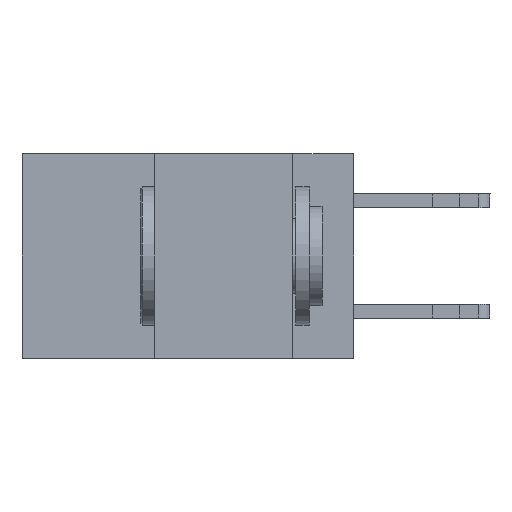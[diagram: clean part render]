
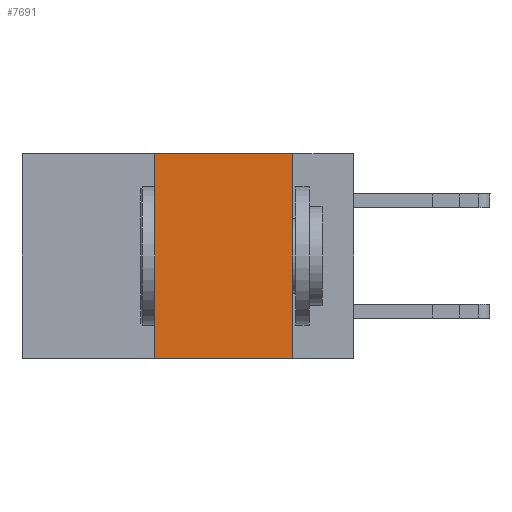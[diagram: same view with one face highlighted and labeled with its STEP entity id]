
A CAD part, left-side view. The second image highlights one B-rep face of the part: STEP entity #7691.
In plain terms, the highlighted planar face has unit normal (-1, 0, 0).
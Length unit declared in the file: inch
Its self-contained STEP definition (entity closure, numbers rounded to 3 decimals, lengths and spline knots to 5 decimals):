
#512 = ORIENTED_EDGE ( 'NONE', *, *, #19916, .T. ) ;
#873 = VERTEX_POINT ( 'NONE', #5513 ) ;
#1558 = LINE ( 'NONE', #6928, #5546 ) ;
#1617 = VECTOR ( 'NONE', #9361, 39.37008 ) ;
#2016 = CARTESIAN_POINT ( 'NONE',  ( 0., 0.36, 0. ) ) ;
#2314 = VERTEX_POINT ( 'NONE', #3720 ) ;
#3064 = DIRECTION ( 'NONE',  ( 0., -1., 0. ) ) ;
#3720 = CARTESIAN_POINT ( 'NONE',  ( 0., 0.36, 0. ) ) ;
#4131 = PLANE ( 'NONE',  #12934 ) ;
#5078 = VERTEX_POINT ( 'NONE', #23108 ) ;
#5513 = CARTESIAN_POINT ( 'NONE',  ( 0., 0.11, -0.37 ) ) ;
#5546 = VECTOR ( 'NONE', #3064, 39.37008 ) ;
#6098 = DIRECTION ( 'NONE',  ( 1., 0., 0. ) ) ;
#6928 = CARTESIAN_POINT ( 'NONE',  ( 0., 0.6, -0.37 ) ) ;
#7691 = ADVANCED_FACE ( 'NONE', ( #10161 ), #4131, .F. ) ;
#8026 = LINE ( 'NONE', #15121, #1617 ) ;
#8850 = CARTESIAN_POINT ( 'NONE',  ( 0., 0.6, 0. ) ) ;
#9095 = ORIENTED_EDGE ( 'NONE', *, *, #25102, .F. ) ;
#9361 = DIRECTION ( 'NONE',  ( 0., 0., -1. ) ) ;
#10161 = FACE_OUTER_BOUND ( 'NONE', #15885, .T. ) ;
#12934 = AXIS2_PLACEMENT_3D ( 'NONE', #23488, #6098, #19677 ) ;
#14744 = LINE ( 'NONE', #2016, #20527 ) ;
#15121 = CARTESIAN_POINT ( 'NONE',  ( 0., 0.11, 0. ) ) ;
#15437 = ORIENTED_EDGE ( 'NONE', *, *, #22059, .F. ) ;
#15885 = EDGE_LOOP ( 'NONE', ( #9095, #15437, #22146, #512 ) ) ;
#17593 = DIRECTION ( 'NONE',  ( 0., 0., 1. ) ) ;
#19677 = DIRECTION ( 'NONE',  ( 0., 0., -1. ) ) ;
#19916 = EDGE_CURVE ( 'NONE', #5078, #873, #1558, .T. ) ;
#20527 = VECTOR ( 'NONE', #17593, 39.37008 ) ;
#21816 = VERTEX_POINT ( 'NONE', #23710 ) ;
#22059 = EDGE_CURVE ( 'NONE', #2314, #21816, #23948, .T. ) ;
#22146 = ORIENTED_EDGE ( 'NONE', *, *, #24328, .F. ) ;
#22521 = DIRECTION ( 'NONE',  ( 0., -1., 0. ) ) ;
#22731 = VECTOR ( 'NONE', #22521, 39.37008 ) ;
#23108 = CARTESIAN_POINT ( 'NONE',  ( 0., 0.36, -0.37 ) ) ;
#23488 = CARTESIAN_POINT ( 'NONE',  ( 0., 0.6, 0. ) ) ;
#23710 = CARTESIAN_POINT ( 'NONE',  ( 0., 0.11, 0. ) ) ;
#23948 = LINE ( 'NONE', #8850, #22731 ) ;
#24328 = EDGE_CURVE ( 'NONE', #5078, #2314, #14744, .T. ) ;
#25102 = EDGE_CURVE ( 'NONE', #21816, #873, #8026, .T. ) ;
